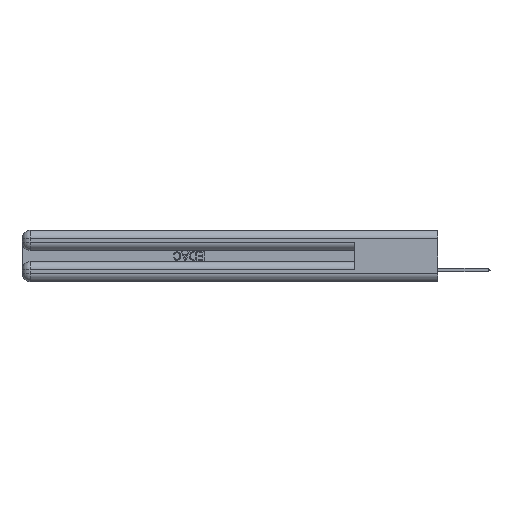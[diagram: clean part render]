
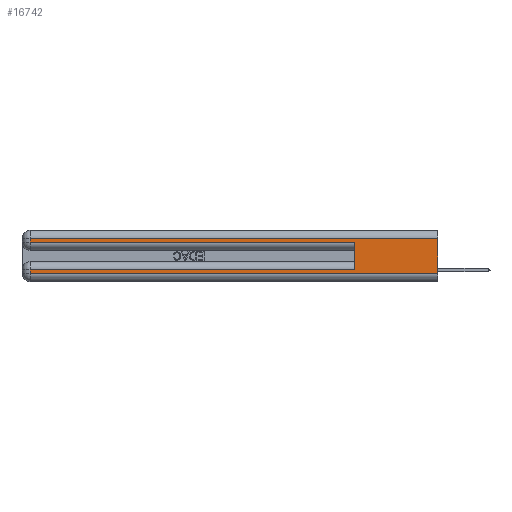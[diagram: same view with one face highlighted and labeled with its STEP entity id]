
A CAD part, left-side view. The second image highlights one B-rep face of the part: STEP entity #16742.
In plain terms, the highlighted planar face has unit normal (-1, 0, 0).
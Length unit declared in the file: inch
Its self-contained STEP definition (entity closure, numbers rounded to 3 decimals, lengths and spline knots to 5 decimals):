
#1326 = EDGE_CURVE ( 'NONE', #38948, #43908, #39478, .T. ) ;
#2917 = EDGE_CURVE ( 'NONE', #18851, #8394, #38062, .T. ) ;
#4378 = CARTESIAN_POINT ( 'NONE',  ( 0., 0., 0.06 ) ) ;
#5284 = VECTOR ( 'NONE', #44538, 39.37008 ) ;
#5918 = DIRECTION ( 'NONE',  ( 0., 1., 0. ) ) ;
#6125 = DIRECTION ( 'NONE',  ( 0., 0., -1. ) ) ;
#6527 = DIRECTION ( 'NONE',  ( 0., -1., 0. ) ) ;
#6898 = CARTESIAN_POINT ( 'NONE',  ( 0., 0., 0.285 ) ) ;
#7463 = VECTOR ( 'NONE', #5918, 39.37008 ) ;
#7517 = CARTESIAN_POINT ( 'NONE',  ( 0., 2.94, 0.37 ) ) ;
#7670 = DIRECTION ( 'NONE',  ( 0., -1., 0. ) ) ;
#8394 = VERTEX_POINT ( 'NONE', #4378 ) ;
#12030 = DIRECTION ( 'NONE',  ( 0., 1., 0. ) ) ;
#12078 = DIRECTION ( 'NONE',  ( 0., 0., -1. ) ) ;
#12782 = VECTOR ( 'NONE', #12030, 39.37008 ) ;
#13729 = ORIENTED_EDGE ( 'NONE', *, *, #43460, .T. ) ;
#16427 = ORIENTED_EDGE ( 'NONE', *, *, #35360, .T. ) ;
#16538 = EDGE_CURVE ( 'NONE', #42476, #41442, #53243, .T. ) ;
#16742 = ADVANCED_FACE ( 'NONE', ( #50674 ), #26482, .F. ) ;
#16839 = CARTESIAN_POINT ( 'NONE',  ( 0., 0.6, 0.085 ) ) ;
#16916 = VERTEX_POINT ( 'NONE', #50308 ) ;
#17384 = VECTOR ( 'NONE', #7670, 39.37008 ) ;
#18174 = DIRECTION ( 'NONE',  ( 1., 0., 0. ) ) ;
#18565 = LINE ( 'NONE', #36759, #12782 ) ;
#18851 = VERTEX_POINT ( 'NONE', #31903 ) ;
#19401 = CARTESIAN_POINT ( 'NONE',  ( 0., 0., 0.31 ) ) ;
#19977 = DIRECTION ( 'NONE',  ( 0., 0., -1. ) ) ;
#20239 = ORIENTED_EDGE ( 'NONE', *, *, #1326, .T. ) ;
#20438 = CARTESIAN_POINT ( 'NONE',  ( 0., 0., 0.06 ) ) ;
#20843 = VERTEX_POINT ( 'NONE', #19401 ) ;
#21776 = VECTOR ( 'NONE', #12078, 39.37008 ) ;
#22725 = ORIENTED_EDGE ( 'NONE', *, *, #2917, .T. ) ;
#26482 = PLANE ( 'NONE',  #45685 ) ;
#27985 = VECTOR ( 'NONE', #47672, 39.37008 ) ;
#30558 = LINE ( 'NONE', #41950, #36378 ) ;
#31267 = ORIENTED_EDGE ( 'NONE', *, *, #47094, .T. ) ;
#31903 = CARTESIAN_POINT ( 'NONE',  ( 0., 2.94, 0.06 ) ) ;
#34084 = CARTESIAN_POINT ( 'NONE',  ( 0., 0.6, 0.285 ) ) ;
#34461 = CARTESIAN_POINT ( 'NONE',  ( 0., 2.94, 0.285 ) ) ;
#35360 = EDGE_CURVE ( 'NONE', #43908, #41442, #51620, .T. ) ;
#36378 = VECTOR ( 'NONE', #19977, 39.37008 ) ;
#36759 = CARTESIAN_POINT ( 'NONE',  ( 0., 0., 0.31 ) ) ;
#37494 = CARTESIAN_POINT ( 'NONE',  ( 0., 0., 0.37 ) ) ;
#38062 = LINE ( 'NONE', #20438, #17384 ) ;
#38948 = VERTEX_POINT ( 'NONE', #47398 ) ;
#39478 = LINE ( 'NONE', #7517, #5284 ) ;
#41442 = VERTEX_POINT ( 'NONE', #34084 ) ;
#41950 = CARTESIAN_POINT ( 'NONE',  ( 0., 2.94, 0.37 ) ) ;
#42476 = VERTEX_POINT ( 'NONE', #16839 ) ;
#43109 = CARTESIAN_POINT ( 'NONE',  ( 0., 0., 0.085 ) ) ;
#43284 = EDGE_LOOP ( 'NONE', ( #46228, #49672, #20239, #16427, #50040, #31267, #13729, #22725 ) ) ;
#43460 = EDGE_CURVE ( 'NONE', #16916, #18851, #30558, .T. ) ;
#43908 = VERTEX_POINT ( 'NONE', #34461 ) ;
#44538 = DIRECTION ( 'NONE',  ( 0., 0., -1. ) ) ;
#45685 = AXIS2_PLACEMENT_3D ( 'NONE', #47260, #18174, #6125 ) ;
#45706 = LINE ( 'NONE', #37494, #21776 ) ;
#46100 = EDGE_CURVE ( 'NONE', #20843, #8394, #45706, .T. ) ;
#46228 = ORIENTED_EDGE ( 'NONE', *, *, #46100, .F. ) ;
#47094 = EDGE_CURVE ( 'NONE', #42476, #16916, #48784, .T. ) ;
#47260 = CARTESIAN_POINT ( 'NONE',  ( 0., 0., 0.37 ) ) ;
#47398 = CARTESIAN_POINT ( 'NONE',  ( 0., 2.94, 0.31 ) ) ;
#47672 = DIRECTION ( 'NONE',  ( 0., 0., 1. ) ) ;
#47844 = CARTESIAN_POINT ( 'NONE',  ( 0., 0.6, 0.145 ) ) ;
#48784 = LINE ( 'NONE', #43109, #7463 ) ;
#49672 = ORIENTED_EDGE ( 'NONE', *, *, #52184, .T. ) ;
#49678 = VECTOR ( 'NONE', #6527, 39.37008 ) ;
#50040 = ORIENTED_EDGE ( 'NONE', *, *, #16538, .F. ) ;
#50308 = CARTESIAN_POINT ( 'NONE',  ( 0., 2.94, 0.085 ) ) ;
#50674 = FACE_OUTER_BOUND ( 'NONE', #43284, .T. ) ;
#51620 = LINE ( 'NONE', #6898, #49678 ) ;
#52184 = EDGE_CURVE ( 'NONE', #20843, #38948, #18565, .T. ) ;
#53243 = LINE ( 'NONE', #47844, #27985 ) ;
